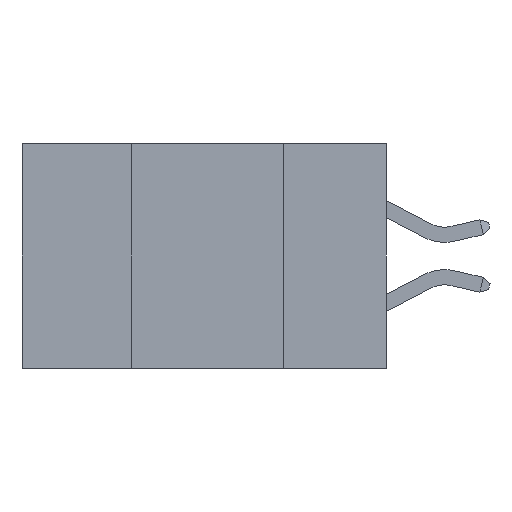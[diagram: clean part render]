
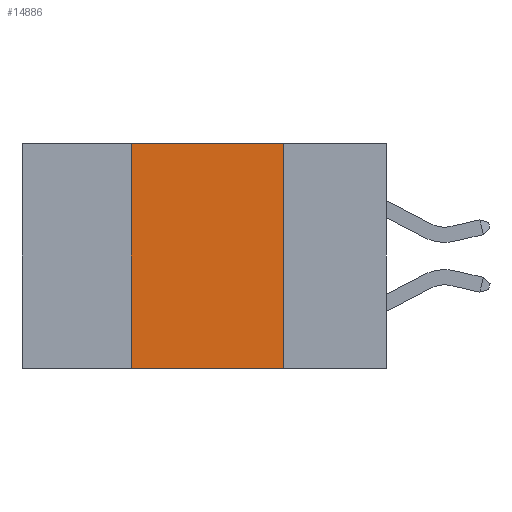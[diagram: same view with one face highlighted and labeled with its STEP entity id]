
A CAD part, left-side view. The second image highlights one B-rep face of the part: STEP entity #14886.
In plain terms, the highlighted planar face has unit normal (-1, 0, 0).
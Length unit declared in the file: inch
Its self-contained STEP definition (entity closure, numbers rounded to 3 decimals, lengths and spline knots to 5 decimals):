
#314 = VERTEX_POINT ( 'NONE', #19622 ) ;
#933 = VECTOR ( 'NONE', #5076, 39.37008 ) ;
#1825 = CARTESIAN_POINT ( 'NONE',  ( 0., 0.6, 0. ) ) ;
#2717 = PLANE ( 'NONE',  #16260 ) ;
#3483 = LINE ( 'NONE', #7392, #17331 ) ;
#5076 = DIRECTION ( 'NONE',  ( 0., 0., -1. ) ) ;
#6127 = LINE ( 'NONE', #1825, #10961 ) ;
#7392 = CARTESIAN_POINT ( 'NONE',  ( 0., 0.6, -0.37 ) ) ;
#7836 = VERTEX_POINT ( 'NONE', #10109 ) ;
#8038 = ORIENTED_EDGE ( 'NONE', *, *, #12426, .F. ) ;
#8481 = ORIENTED_EDGE ( 'NONE', *, *, #18880, .F. ) ;
#8502 = VECTOR ( 'NONE', #13848, 39.37008 ) ;
#8780 = EDGE_CURVE ( 'NONE', #7836, #22851, #6127, .T. ) ;
#8954 = VERTEX_POINT ( 'NONE', #11437 ) ;
#10014 = DIRECTION ( 'NONE',  ( 1., 0., 0. ) ) ;
#10109 = CARTESIAN_POINT ( 'NONE',  ( 0., 0.42, 0. ) ) ;
#10845 = EDGE_LOOP ( 'NONE', ( #8038, #19190, #8481, #19699 ) ) ;
#10961 = VECTOR ( 'NONE', #12672, 39.37008 ) ;
#11046 = DIRECTION ( 'NONE',  ( 0., -1., 0. ) ) ;
#11437 = CARTESIAN_POINT ( 'NONE',  ( 0., 0.17, -0.37 ) ) ;
#12426 = EDGE_CURVE ( 'NONE', #22851, #8954, #14836, .T. ) ;
#12672 = DIRECTION ( 'NONE',  ( 0., -1., 0. ) ) ;
#13848 = DIRECTION ( 'NONE',  ( 0., 0., 1. ) ) ;
#13864 = LINE ( 'NONE', #17444, #8502 ) ;
#14836 = LINE ( 'NONE', #17702, #933 ) ;
#14886 = ADVANCED_FACE ( 'NONE', ( #18407 ), #2717, .F. ) ;
#16260 = AXIS2_PLACEMENT_3D ( 'NONE', #20774, #10014, #22597 ) ;
#16930 = EDGE_CURVE ( 'NONE', #314, #8954, #3483, .T. ) ;
#17331 = VECTOR ( 'NONE', #11046, 39.37008 ) ;
#17444 = CARTESIAN_POINT ( 'NONE',  ( 0., 0.42, -0.37 ) ) ;
#17702 = CARTESIAN_POINT ( 'NONE',  ( 0., 0.17, -0.37 ) ) ;
#18407 = FACE_OUTER_BOUND ( 'NONE', #10845, .T. ) ;
#18880 = EDGE_CURVE ( 'NONE', #314, #7836, #13864, .T. ) ;
#19190 = ORIENTED_EDGE ( 'NONE', *, *, #8780, .F. ) ;
#19622 = CARTESIAN_POINT ( 'NONE',  ( 0., 0.42, -0.37 ) ) ;
#19699 = ORIENTED_EDGE ( 'NONE', *, *, #16930, .T. ) ;
#19860 = CARTESIAN_POINT ( 'NONE',  ( 0., 0.17, 0. ) ) ;
#20774 = CARTESIAN_POINT ( 'NONE',  ( 0., 0.6, 0. ) ) ;
#22597 = DIRECTION ( 'NONE',  ( 0., 0., -1. ) ) ;
#22851 = VERTEX_POINT ( 'NONE', #19860 ) ;
